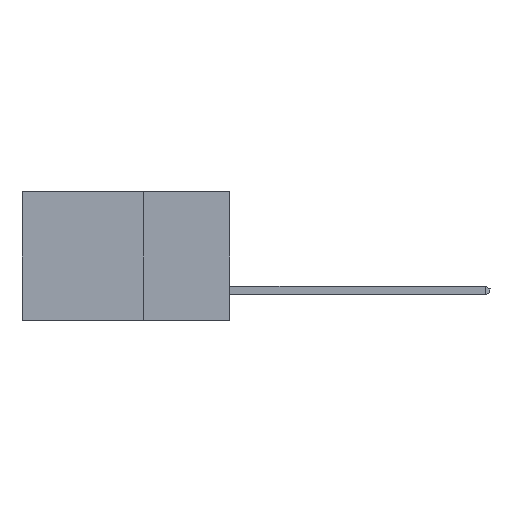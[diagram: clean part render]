
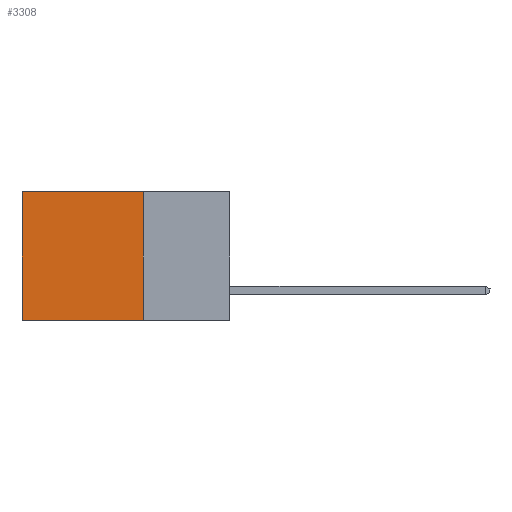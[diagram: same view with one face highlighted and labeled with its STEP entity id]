
A CAD part, left-side view. The second image highlights one B-rep face of the part: STEP entity #3308.
In plain terms, the highlighted planar face has unit normal (-1, 0, 0).
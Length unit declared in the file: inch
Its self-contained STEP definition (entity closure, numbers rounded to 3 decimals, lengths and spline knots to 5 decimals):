
#124 = CARTESIAN_POINT ( 'NONE',  ( 0.2615, 0.25, 0. ) ) ;
#1121 = FACE_OUTER_BOUND ( 'NONE', #11788, .T. ) ;
#1476 = LINE ( 'NONE', #124, #5204 ) ;
#1507 = ORIENTED_EDGE ( 'NONE', *, *, #5812, .F. ) ;
#2306 = EDGE_CURVE ( 'NONE', #11283, #9947, #1476, .T. ) ;
#2415 = ORIENTED_EDGE ( 'NONE', *, *, #2306, .T. ) ;
#3308 = ADVANCED_FACE ( 'NONE', ( #1121 ), #9492, .F. ) ;
#3338 = DIRECTION ( 'NONE',  ( 0., 0., -1. ) ) ;
#4344 = LINE ( 'NONE', #14258, #11895 ) ;
#4407 = VECTOR ( 'NONE', #10663, 39.37008 ) ;
#4816 = EDGE_CURVE ( 'NONE', #11283, #7410, #4344, .T. ) ;
#5204 = VECTOR ( 'NONE', #6949, 39.37008 ) ;
#5649 = CARTESIAN_POINT ( 'NONE',  ( 0.2615, 0.25, -0.37 ) ) ;
#5719 = DIRECTION ( 'NONE',  ( 0., 0., -1. ) ) ;
#5812 = EDGE_CURVE ( 'NONE', #7410, #7815, #8054, .T. ) ;
#6949 = DIRECTION ( 'NONE',  ( 0., 1., 0. ) ) ;
#7410 = VERTEX_POINT ( 'NONE', #5649 ) ;
#7815 = VERTEX_POINT ( 'NONE', #8583 ) ;
#8054 = LINE ( 'NONE', #10840, #4407 ) ;
#8583 = CARTESIAN_POINT ( 'NONE',  ( 0.2615, 0.6, -0.37 ) ) ;
#8921 = CARTESIAN_POINT ( 'NONE',  ( 0.2615, 0.6, -0.37 ) ) ;
#9492 = PLANE ( 'NONE',  #13224 ) ;
#9580 = DIRECTION ( 'NONE',  ( 0., 0., -1. ) ) ;
#9947 = VERTEX_POINT ( 'NONE', #11235 ) ;
#10185 = LINE ( 'NONE', #8921, #12791 ) ;
#10653 = DIRECTION ( 'NONE',  ( 1., 0., 0. ) ) ;
#10663 = DIRECTION ( 'NONE',  ( 0., 1., 0. ) ) ;
#10840 = CARTESIAN_POINT ( 'NONE',  ( 0.2615, 0.25, -0.37 ) ) ;
#10991 = CARTESIAN_POINT ( 'NONE',  ( 0.2615, 0.25, 0. ) ) ;
#11235 = CARTESIAN_POINT ( 'NONE',  ( 0.2615, 0.6, 0. ) ) ;
#11283 = VERTEX_POINT ( 'NONE', #10991 ) ;
#11788 = EDGE_LOOP ( 'NONE', ( #12195, #1507, #14146, #2415 ) ) ;
#11895 = VECTOR ( 'NONE', #5719, 39.37008 ) ;
#12195 = ORIENTED_EDGE ( 'NONE', *, *, #17110, .T. ) ;
#12791 = VECTOR ( 'NONE', #3338, 39.37008 ) ;
#13224 = AXIS2_PLACEMENT_3D ( 'NONE', #16511, #10653, #9580 ) ;
#14146 = ORIENTED_EDGE ( 'NONE', *, *, #4816, .F. ) ;
#14258 = CARTESIAN_POINT ( 'NONE',  ( 0.2615, 0.25, -0.37 ) ) ;
#16511 = CARTESIAN_POINT ( 'NONE',  ( 0.2615, 0.25, -0.37 ) ) ;
#17110 = EDGE_CURVE ( 'NONE', #9947, #7815, #10185, .T. ) ;
